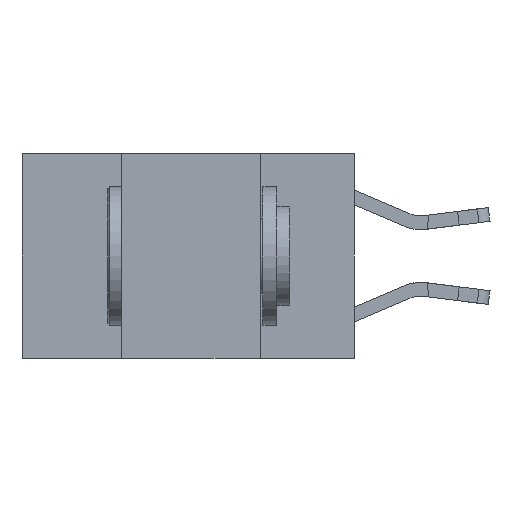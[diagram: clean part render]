
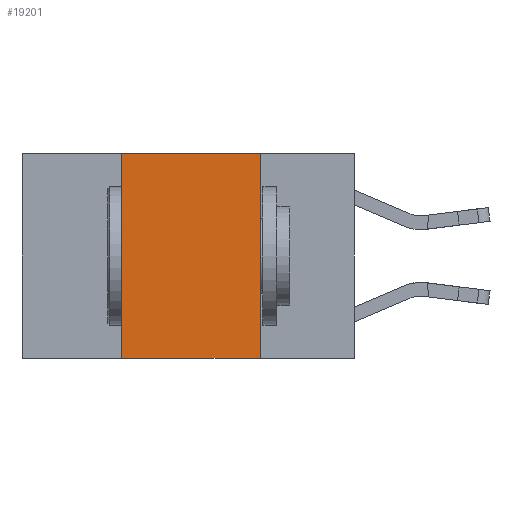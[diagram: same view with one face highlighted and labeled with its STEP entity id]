
A CAD part, left-side view. The second image highlights one B-rep face of the part: STEP entity #19201.
In plain terms, the highlighted planar face has unit normal (-1, 0, 0).
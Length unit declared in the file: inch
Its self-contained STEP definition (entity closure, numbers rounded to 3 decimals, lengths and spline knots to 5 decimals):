
#663 = CARTESIAN_POINT ( 'NONE',  ( 0., 0.42, 0. ) ) ;
#6611 = DIRECTION ( 'NONE',  ( 0., 0., -1. ) ) ;
#7214 = EDGE_CURVE ( 'NONE', #22636, #11507, #25708, .T. ) ;
#7745 = AXIS2_PLACEMENT_3D ( 'NONE', #16428, #16941, #6611 ) ;
#7753 = CARTESIAN_POINT ( 'NONE',  ( 0., 0.6, 0. ) ) ;
#7899 = VECTOR ( 'NONE', #10609, 39.37008 ) ;
#8419 = CARTESIAN_POINT ( 'NONE',  ( 0., 0.42, 0. ) ) ;
#8775 = LINE ( 'NONE', #16770, #22355 ) ;
#10609 = DIRECTION ( 'NONE',  ( 0., 0., -1. ) ) ;
#11507 = VERTEX_POINT ( 'NONE', #15732 ) ;
#11641 = ORIENTED_EDGE ( 'NONE', *, *, #23184, .F. ) ;
#11914 = VECTOR ( 'NONE', #13767, 39.37008 ) ;
#12733 = VERTEX_POINT ( 'NONE', #19527 ) ;
#13346 = ORIENTED_EDGE ( 'NONE', *, *, #7214, .F. ) ;
#13767 = DIRECTION ( 'NONE',  ( 0., -1., 0. ) ) ;
#14283 = LINE ( 'NONE', #18457, #7899 ) ;
#14451 = CARTESIAN_POINT ( 'NONE',  ( 0., 0.17, -0.37 ) ) ;
#14817 = VECTOR ( 'NONE', #22675, 39.37008 ) ;
#15732 = CARTESIAN_POINT ( 'NONE',  ( 0., 0.17, 0. ) ) ;
#15915 = ORIENTED_EDGE ( 'NONE', *, *, #16657, .F. ) ;
#16428 = CARTESIAN_POINT ( 'NONE',  ( 0., 0.6, 0. ) ) ;
#16509 = LINE ( 'NONE', #663, #14817 ) ;
#16657 = EDGE_CURVE ( 'NONE', #12733, #22636, #16509, .T. ) ;
#16762 = EDGE_CURVE ( 'NONE', #12733, #23967, #8775, .T. ) ;
#16770 = CARTESIAN_POINT ( 'NONE',  ( 0., 0.6, -0.37 ) ) ;
#16941 = DIRECTION ( 'NONE',  ( 1., 0., 0. ) ) ;
#18252 = ORIENTED_EDGE ( 'NONE', *, *, #16762, .T. ) ;
#18457 = CARTESIAN_POINT ( 'NONE',  ( 0., 0.17, 0. ) ) ;
#19201 = ADVANCED_FACE ( 'NONE', ( #22988 ), #20736, .F. ) ;
#19527 = CARTESIAN_POINT ( 'NONE',  ( 0., 0.42, -0.37 ) ) ;
#20736 = PLANE ( 'NONE',  #7745 ) ;
#22355 = VECTOR ( 'NONE', #24767, 39.37008 ) ;
#22636 = VERTEX_POINT ( 'NONE', #8419 ) ;
#22675 = DIRECTION ( 'NONE',  ( 0., 0., 1. ) ) ;
#22988 = FACE_OUTER_BOUND ( 'NONE', #24931, .T. ) ;
#23184 = EDGE_CURVE ( 'NONE', #11507, #23967, #14283, .T. ) ;
#23967 = VERTEX_POINT ( 'NONE', #14451 ) ;
#24767 = DIRECTION ( 'NONE',  ( 0., -1., 0. ) ) ;
#24931 = EDGE_LOOP ( 'NONE', ( #11641, #13346, #15915, #18252 ) ) ;
#25708 = LINE ( 'NONE', #7753, #11914 ) ;
